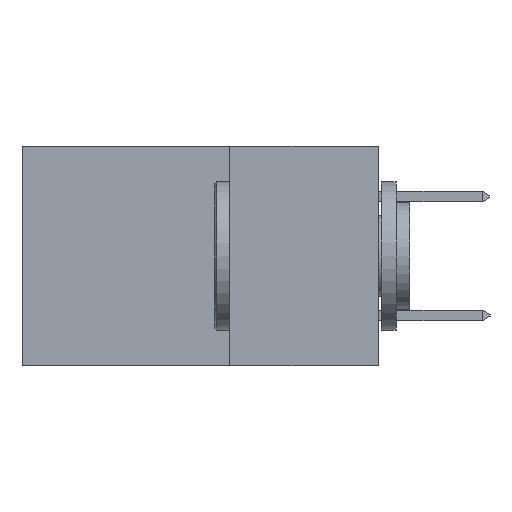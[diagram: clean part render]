
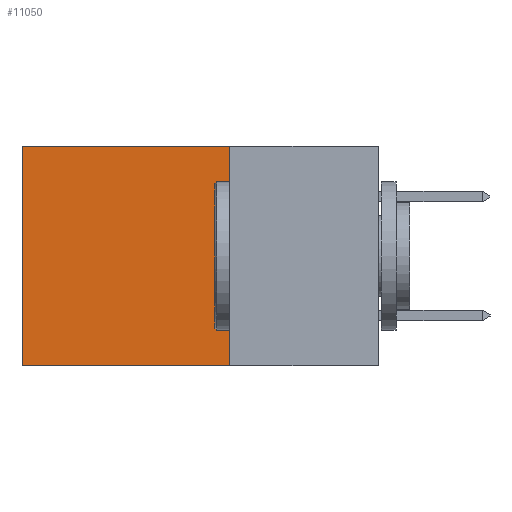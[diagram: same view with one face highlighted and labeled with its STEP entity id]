
A CAD part, left-side view. The second image highlights one B-rep face of the part: STEP entity #11050.
In plain terms, the highlighted planar face has unit normal (-1, 0, 0).
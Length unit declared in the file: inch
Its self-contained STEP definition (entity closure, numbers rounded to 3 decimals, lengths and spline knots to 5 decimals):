
#19 = FACE_OUTER_BOUND ( 'NONE', #5199, .T. ) ;
#559 = DIRECTION ( 'NONE',  ( 0., 0., -1. ) ) ;
#768 = VERTEX_POINT ( 'NONE', #10273 ) ;
#1408 = CARTESIAN_POINT ( 'NONE',  ( 0.2615, 0.6, -0.37 ) ) ;
#1868 = CARTESIAN_POINT ( 'NONE',  ( 0.2615, 0.25, 0. ) ) ;
#1962 = ORIENTED_EDGE ( 'NONE', *, *, #10330, .T. ) ;
#2142 = AXIS2_PLACEMENT_3D ( 'NONE', #11028, #5927, #559 ) ;
#2200 = ORIENTED_EDGE ( 'NONE', *, *, #8822, .F. ) ;
#2523 = EDGE_CURVE ( 'NONE', #11025, #8125, #5836, .T. ) ;
#2558 = VERTEX_POINT ( 'NONE', #10749 ) ;
#2588 = DIRECTION ( 'NONE',  ( 0., 1., 0. ) ) ;
#2601 = CARTESIAN_POINT ( 'NONE',  ( 0.2615, 0.6, 0. ) ) ;
#2886 = DIRECTION ( 'NONE',  ( 0., 1., 0. ) ) ;
#2919 = LINE ( 'NONE', #3838, #9883 ) ;
#3788 = ORIENTED_EDGE ( 'NONE', *, *, #2523, .T. ) ;
#3834 = ORIENTED_EDGE ( 'NONE', *, *, #9877, .F. ) ;
#3838 = CARTESIAN_POINT ( 'NONE',  ( 0.2615, 0.25, -0.37 ) ) ;
#5044 = PLANE ( 'NONE',  #2142 ) ;
#5199 = EDGE_LOOP ( 'NONE', ( #1962, #2200, #3834, #3788 ) ) ;
#5276 = LINE ( 'NONE', #1408, #7299 ) ;
#5836 = LINE ( 'NONE', #1868, #7576 ) ;
#5927 = DIRECTION ( 'NONE',  ( 1., 0., 0. ) ) ;
#7299 = VECTOR ( 'NONE', #11039, 39.37008 ) ;
#7576 = VECTOR ( 'NONE', #2886, 39.37008 ) ;
#7839 = CARTESIAN_POINT ( 'NONE',  ( 0.2615, 0.25, -0.37 ) ) ;
#8125 = VERTEX_POINT ( 'NONE', #2601 ) ;
#8427 = CARTESIAN_POINT ( 'NONE',  ( 0.2615, 0.25, 0. ) ) ;
#8660 = LINE ( 'NONE', #7839, #10182 ) ;
#8822 = EDGE_CURVE ( 'NONE', #2558, #768, #8660, .T. ) ;
#9015 = DIRECTION ( 'NONE',  ( 0., 0., -1. ) ) ;
#9877 = EDGE_CURVE ( 'NONE', #11025, #2558, #2919, .T. ) ;
#9883 = VECTOR ( 'NONE', #9015, 39.37008 ) ;
#10182 = VECTOR ( 'NONE', #2588, 39.37008 ) ;
#10273 = CARTESIAN_POINT ( 'NONE',  ( 0.2615, 0.6, -0.37 ) ) ;
#10330 = EDGE_CURVE ( 'NONE', #8125, #768, #5276, .T. ) ;
#10749 = CARTESIAN_POINT ( 'NONE',  ( 0.2615, 0.25, -0.37 ) ) ;
#11025 = VERTEX_POINT ( 'NONE', #8427 ) ;
#11028 = CARTESIAN_POINT ( 'NONE',  ( 0.2615, 0.25, -0.37 ) ) ;
#11039 = DIRECTION ( 'NONE',  ( 0., 0., -1. ) ) ;
#11050 = ADVANCED_FACE ( 'NONE', ( #19 ), #5044, .F. ) ;
